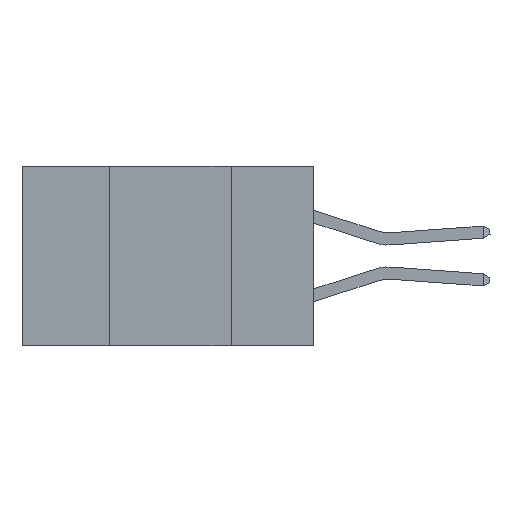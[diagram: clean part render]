
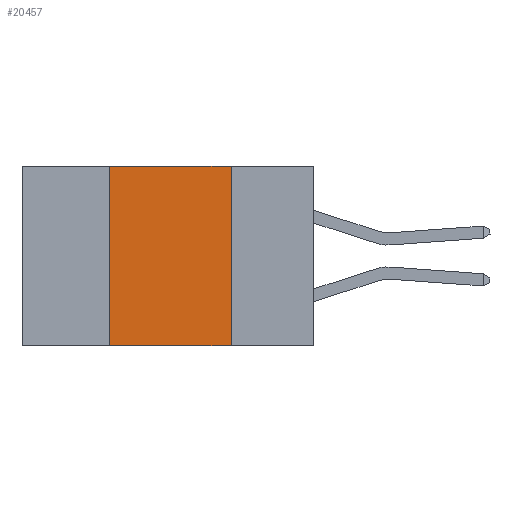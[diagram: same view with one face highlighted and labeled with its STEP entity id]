
A CAD part, left-side view. The second image highlights one B-rep face of the part: STEP entity #20457.
In plain terms, the highlighted planar face has unit normal (-1, 0, 0).
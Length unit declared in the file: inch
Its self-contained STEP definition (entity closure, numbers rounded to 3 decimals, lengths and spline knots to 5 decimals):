
#1236 = EDGE_CURVE ( 'NONE', #11716, #12444, #17022, .T. ) ;
#2242 = CARTESIAN_POINT ( 'NONE',  ( 0., 0.42, 0. ) ) ;
#2303 = PLANE ( 'NONE',  #17661 ) ;
#2397 = DIRECTION ( 'NONE',  ( 0., -1., 0. ) ) ;
#2524 = DIRECTION ( 'NONE',  ( 0., 0., -1. ) ) ;
#3874 = ORIENTED_EDGE ( 'NONE', *, *, #14102, .F. ) ;
#4478 = EDGE_LOOP ( 'NONE', ( #17417, #3874, #18927, #13368 ) ) ;
#5531 = VERTEX_POINT ( 'NONE', #11765 ) ;
#7413 = FACE_OUTER_BOUND ( 'NONE', #4478, .T. ) ;
#7926 = EDGE_CURVE ( 'NONE', #11716, #17172, #10203, .T. ) ;
#9693 = EDGE_CURVE ( 'NONE', #5531, #17172, #13323, .T. ) ;
#10203 = LINE ( 'NONE', #16576, #14281 ) ;
#10561 = CARTESIAN_POINT ( 'NONE',  ( 0., 0.42, 0. ) ) ;
#10586 = CARTESIAN_POINT ( 'NONE',  ( 0., 0.42, -0.37 ) ) ;
#11716 = VERTEX_POINT ( 'NONE', #10586 ) ;
#11765 = CARTESIAN_POINT ( 'NONE',  ( 0., 0.17, 0. ) ) ;
#11973 = CARTESIAN_POINT ( 'NONE',  ( 0., 0.17, 0. ) ) ;
#12444 = VERTEX_POINT ( 'NONE', #2242 ) ;
#13196 = VECTOR ( 'NONE', #19451, 39.37008 ) ;
#13287 = CARTESIAN_POINT ( 'NONE',  ( 0., 0.6, 0. ) ) ;
#13323 = LINE ( 'NONE', #11973, #18829 ) ;
#13368 = ORIENTED_EDGE ( 'NONE', *, *, #7926, .T. ) ;
#13456 = CARTESIAN_POINT ( 'NONE',  ( 0., 0.6, 0. ) ) ;
#13782 = DIRECTION ( 'NONE',  ( 0., 0., 1. ) ) ;
#14102 = EDGE_CURVE ( 'NONE', #12444, #5531, #17271, .T. ) ;
#14281 = VECTOR ( 'NONE', #2397, 39.37008 ) ;
#16053 = VECTOR ( 'NONE', #13782, 39.37008 ) ;
#16310 = CARTESIAN_POINT ( 'NONE',  ( 0., 0.17, -0.37 ) ) ;
#16576 = CARTESIAN_POINT ( 'NONE',  ( 0., 0.6, -0.37 ) ) ;
#17022 = LINE ( 'NONE', #10561, #16053 ) ;
#17172 = VERTEX_POINT ( 'NONE', #16310 ) ;
#17271 = LINE ( 'NONE', #13287, #13196 ) ;
#17417 = ORIENTED_EDGE ( 'NONE', *, *, #9693, .F. ) ;
#17661 = AXIS2_PLACEMENT_3D ( 'NONE', #13456, #19822, #2524 ) ;
#18829 = VECTOR ( 'NONE', #19784, 39.37008 ) ;
#18927 = ORIENTED_EDGE ( 'NONE', *, *, #1236, .F. ) ;
#19451 = DIRECTION ( 'NONE',  ( 0., -1., 0. ) ) ;
#19784 = DIRECTION ( 'NONE',  ( 0., 0., -1. ) ) ;
#19822 = DIRECTION ( 'NONE',  ( 1., 0., 0. ) ) ;
#20457 = ADVANCED_FACE ( 'NONE', ( #7413 ), #2303, .F. ) ;
